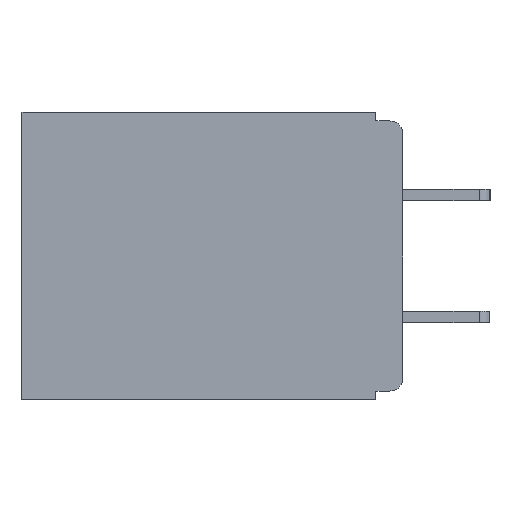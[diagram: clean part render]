
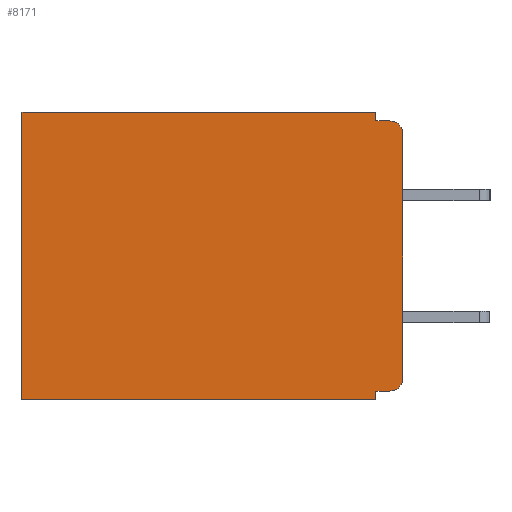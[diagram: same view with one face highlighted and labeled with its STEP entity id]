
A CAD part, left-side view. The second image highlights one B-rep face of the part: STEP entity #8171.
In plain terms, the highlighted planar face has unit normal (-1, 0, 0).
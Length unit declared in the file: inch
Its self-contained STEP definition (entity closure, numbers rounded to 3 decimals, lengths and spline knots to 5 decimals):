
#463 = VECTOR ( 'NONE', #15601, 39.37008 ) ;
#582 = ORIENTED_EDGE ( 'NONE', *, *, #2010, .F. ) ;
#979 = CARTESIAN_POINT ( 'NONE',  ( 0.3, 0., -0.33 ) ) ;
#1196 = VERTEX_POINT ( 'NONE', #19614 ) ;
#1291 = DIRECTION ( 'NONE',  ( 0., 0., -1. ) ) ;
#1434 = CARTESIAN_POINT ( 'NONE',  ( 0.3, 0.015, -0.305 ) ) ;
#2010 = EDGE_CURVE ( 'NONE', #12958, #22488, #7463, .T. ) ;
#2311 = ORIENTED_EDGE ( 'NONE', *, *, #19461, .F. ) ;
#2740 = ORIENTED_EDGE ( 'NONE', *, *, #14337, .F. ) ;
#2942 = VERTEX_POINT ( 'NONE', #16860 ) ;
#3013 = EDGE_CURVE ( 'NONE', #28038, #22488, #9353, .T. ) ;
#3615 = EDGE_CURVE ( 'NONE', #10805, #11231, #23317, .T. ) ;
#4040 = DIRECTION ( 'NONE',  ( 0., 0., -1. ) ) ;
#4553 = VERTEX_POINT ( 'NONE', #19533 ) ;
#4562 = AXIS2_PLACEMENT_3D ( 'NONE', #26276, #15864, #26021 ) ;
#4725 = LINE ( 'NONE', #30039, #9905 ) ;
#5056 = EDGE_LOOP ( 'NONE', ( #2311, #31243, #582, #27963, #13032, #31559, #2740, #13235, #32017, #26415 ) ) ;
#5375 = VECTOR ( 'NONE', #29568, 39.37008 ) ;
#5951 = VERTEX_POINT ( 'NONE', #28656 ) ;
#6202 = DIRECTION ( 'NONE',  ( 0., 0., -1. ) ) ;
#7240 = EDGE_CURVE ( 'NONE', #1196, #4553, #4725, .T. ) ;
#7350 = LINE ( 'NONE', #25790, #463 ) ;
#7463 = LINE ( 'NONE', #24248, #27084 ) ;
#7645 = CARTESIAN_POINT ( 'NONE',  ( 0.3, 0.031, -0.01 ) ) ;
#8171 = ADVANCED_FACE ( 'NONE', ( #9428 ), #16361, .F. ) ;
#9186 = VECTOR ( 'NONE', #20161, 39.37008 ) ;
#9353 = CIRCLE ( 'NONE', #4562, 0.015 ) ;
#9428 = FACE_OUTER_BOUND ( 'NONE', #5056, .T. ) ;
#9905 = VECTOR ( 'NONE', #19659, 39.37008 ) ;
#10480 = AXIS2_PLACEMENT_3D ( 'NONE', #1434, #19373, #4040 ) ;
#10805 = VERTEX_POINT ( 'NONE', #17514 ) ;
#11231 = VERTEX_POINT ( 'NONE', #27002 ) ;
#11305 = VECTOR ( 'NONE', #29759, 39.37008 ) ;
#11390 = DIRECTION ( 'NONE',  ( 0., 1., 0. ) ) ;
#11587 = CARTESIAN_POINT ( 'NONE',  ( 0.3, 0.031, 0. ) ) ;
#12041 = CIRCLE ( 'NONE', #10480, 0.015 ) ;
#12435 = CARTESIAN_POINT ( 'NONE',  ( 0.3, 0., 0. ) ) ;
#12536 = CARTESIAN_POINT ( 'NONE',  ( 0.3, 0.015, -0.32 ) ) ;
#12908 = VERTEX_POINT ( 'NONE', #12536 ) ;
#12958 = VERTEX_POINT ( 'NONE', #7645 ) ;
#13032 = ORIENTED_EDGE ( 'NONE', *, *, #28164, .T. ) ;
#13235 = ORIENTED_EDGE ( 'NONE', *, *, #3615, .F. ) ;
#14337 = EDGE_CURVE ( 'NONE', #11231, #4553, #7350, .T. ) ;
#14601 = LINE ( 'NONE', #26762, #28263 ) ;
#15089 = EDGE_CURVE ( 'NONE', #12908, #5951, #12041, .T. ) ;
#15493 = AXIS2_PLACEMENT_3D ( 'NONE', #979, #21457, #6202 ) ;
#15601 = DIRECTION ( 'NONE',  ( 0., 1., 0. ) ) ;
#15864 = DIRECTION ( 'NONE',  ( -1., 0., 0. ) ) ;
#16361 = PLANE ( 'NONE',  #15493 ) ;
#16860 = CARTESIAN_POINT ( 'NONE',  ( 0.3, 0.031, 0. ) ) ;
#17514 = CARTESIAN_POINT ( 'NONE',  ( 0.3, 0.031, -0.32 ) ) ;
#18084 = CARTESIAN_POINT ( 'NONE',  ( 0.3, 0.015, -0.01 ) ) ;
#18960 = LINE ( 'NONE', #11587, #5375 ) ;
#19373 = DIRECTION ( 'NONE',  ( -1., 0., 0. ) ) ;
#19406 = EDGE_CURVE ( 'NONE', #12908, #10805, #14601, .T. ) ;
#19461 = EDGE_CURVE ( 'NONE', #28038, #5951, #26646, .T. ) ;
#19533 = CARTESIAN_POINT ( 'NONE',  ( 0.3, 0.437, -0.33 ) ) ;
#19614 = CARTESIAN_POINT ( 'NONE',  ( 0.3, 0.437, 0. ) ) ;
#19659 = DIRECTION ( 'NONE',  ( 0., 0., -1. ) ) ;
#20161 = DIRECTION ( 'NONE',  ( 0., 1., 0. ) ) ;
#20769 = CARTESIAN_POINT ( 'NONE',  ( 0.3, 0.031, -0.33 ) ) ;
#21457 = DIRECTION ( 'NONE',  ( 1., 0., 0. ) ) ;
#21756 = CARTESIAN_POINT ( 'NONE',  ( 0.3, 0., -0.33 ) ) ;
#22488 = VERTEX_POINT ( 'NONE', #18084 ) ;
#23317 = LINE ( 'NONE', #20769, #11305 ) ;
#23597 = LINE ( 'NONE', #12435, #9186 ) ;
#23939 = DIRECTION ( 'NONE',  ( 0., -1., 0. ) ) ;
#24248 = CARTESIAN_POINT ( 'NONE',  ( 0.3, 0., -0.01 ) ) ;
#25790 = CARTESIAN_POINT ( 'NONE',  ( 0.3, 0., -0.33 ) ) ;
#25822 = VECTOR ( 'NONE', #1291, 39.37008 ) ;
#26021 = DIRECTION ( 'NONE',  ( 0., 0., -1. ) ) ;
#26276 = CARTESIAN_POINT ( 'NONE',  ( 0.3, 0.015, -0.025 ) ) ;
#26415 = ORIENTED_EDGE ( 'NONE', *, *, #15089, .T. ) ;
#26646 = LINE ( 'NONE', #21756, #25822 ) ;
#26762 = CARTESIAN_POINT ( 'NONE',  ( 0.3, 0., -0.32 ) ) ;
#27002 = CARTESIAN_POINT ( 'NONE',  ( 0.3, 0.031, -0.33 ) ) ;
#27084 = VECTOR ( 'NONE', #23939, 39.37008 ) ;
#27963 = ORIENTED_EDGE ( 'NONE', *, *, #31212, .F. ) ;
#28038 = VERTEX_POINT ( 'NONE', #30000 ) ;
#28164 = EDGE_CURVE ( 'NONE', #2942, #1196, #23597, .T. ) ;
#28263 = VECTOR ( 'NONE', #11390, 39.37008 ) ;
#28656 = CARTESIAN_POINT ( 'NONE',  ( 0.3, 0., -0.305 ) ) ;
#29568 = DIRECTION ( 'NONE',  ( 0., 0., -1. ) ) ;
#29759 = DIRECTION ( 'NONE',  ( 0., 0., -1. ) ) ;
#30000 = CARTESIAN_POINT ( 'NONE',  ( 0.3, 0., -0.025 ) ) ;
#30039 = CARTESIAN_POINT ( 'NONE',  ( 0.3, 0.437, -0.33 ) ) ;
#31212 = EDGE_CURVE ( 'NONE', #2942, #12958, #18960, .T. ) ;
#31243 = ORIENTED_EDGE ( 'NONE', *, *, #3013, .T. ) ;
#31559 = ORIENTED_EDGE ( 'NONE', *, *, #7240, .T. ) ;
#32017 = ORIENTED_EDGE ( 'NONE', *, *, #19406, .F. ) ;
